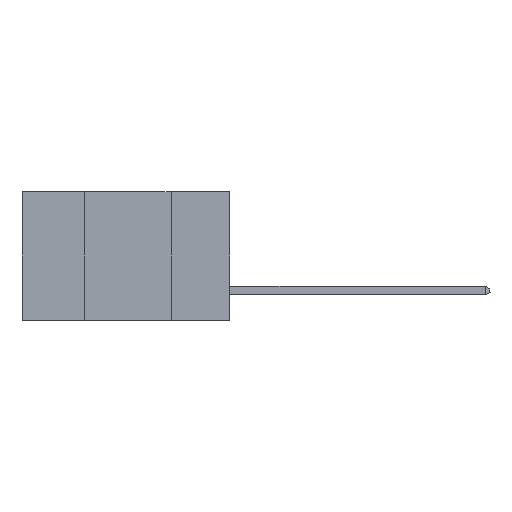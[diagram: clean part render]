
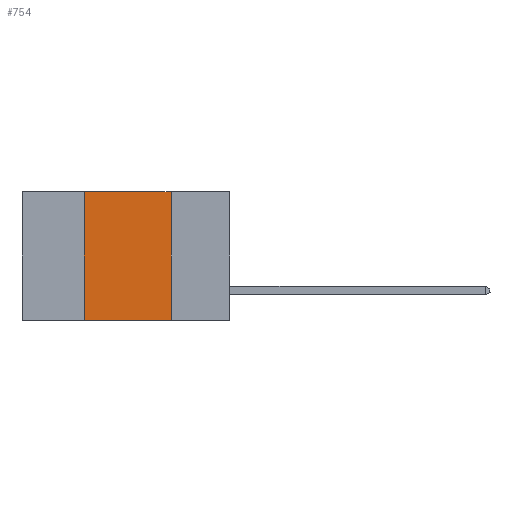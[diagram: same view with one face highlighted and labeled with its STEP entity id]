
A CAD part, left-side view. The second image highlights one B-rep face of the part: STEP entity #754.
In plain terms, the highlighted planar face has unit normal (-1, 0, 0).
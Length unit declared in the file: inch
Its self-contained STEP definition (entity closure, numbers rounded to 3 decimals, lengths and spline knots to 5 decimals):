
#754 = ADVANCED_FACE ( 'NONE', ( #15377 ), #8433, .F. ) ;
#2113 = VECTOR ( 'NONE', #14111, 39.37008 ) ;
#2684 = DIRECTION ( 'NONE',  ( 0., 0., 1. ) ) ;
#4161 = CARTESIAN_POINT ( 'NONE',  ( 0., 0.6, -0.37 ) ) ;
#4231 = CARTESIAN_POINT ( 'NONE',  ( 0., 0.42, 0. ) ) ;
#4242 = LINE ( 'NONE', #9874, #2113 ) ;
#4556 = DIRECTION ( 'NONE',  ( 0., 0., -1. ) ) ;
#5017 = ORIENTED_EDGE ( 'NONE', *, *, #5568, .F. ) ;
#5330 = ORIENTED_EDGE ( 'NONE', *, *, #8817, .F. ) ;
#5568 = EDGE_CURVE ( 'NONE', #24593, #8325, #8588, .T. ) ;
#6742 = DIRECTION ( 'NONE',  ( 1., 0., 0. ) ) ;
#8325 = VERTEX_POINT ( 'NONE', #4231 ) ;
#8433 = PLANE ( 'NONE',  #16339 ) ;
#8588 = LINE ( 'NONE', #8654, #13114 ) ;
#8654 = CARTESIAN_POINT ( 'NONE',  ( 0., 0.42, 0. ) ) ;
#8679 = CARTESIAN_POINT ( 'NONE',  ( 0., 0.6, 0. ) ) ;
#8817 = EDGE_CURVE ( 'NONE', #24569, #12203, #13921, .T. ) ;
#9874 = CARTESIAN_POINT ( 'NONE',  ( 0., 0.6, 0. ) ) ;
#10354 = VECTOR ( 'NONE', #14090, 39.37008 ) ;
#11654 = CARTESIAN_POINT ( 'NONE',  ( 0., 0.17, 0. ) ) ;
#12203 = VERTEX_POINT ( 'NONE', #24895 ) ;
#12506 = ORIENTED_EDGE ( 'NONE', *, *, #19374, .T. ) ;
#13114 = VECTOR ( 'NONE', #2684, 39.37008 ) ;
#13144 = EDGE_LOOP ( 'NONE', ( #5330, #22034, #5017, #12506 ) ) ;
#13921 = LINE ( 'NONE', #11654, #17844 ) ;
#14090 = DIRECTION ( 'NONE',  ( 0., -1., 0. ) ) ;
#14111 = DIRECTION ( 'NONE',  ( 0., -1., 0. ) ) ;
#14818 = CARTESIAN_POINT ( 'NONE',  ( 0., 0.17, 0. ) ) ;
#15377 = FACE_OUTER_BOUND ( 'NONE', #13144, .T. ) ;
#16339 = AXIS2_PLACEMENT_3D ( 'NONE', #8679, #6742, #4556 ) ;
#17844 = VECTOR ( 'NONE', #22907, 39.37008 ) ;
#19374 = EDGE_CURVE ( 'NONE', #24593, #12203, #20639, .T. ) ;
#20002 = EDGE_CURVE ( 'NONE', #8325, #24569, #4242, .T. ) ;
#20639 = LINE ( 'NONE', #4161, #10354 ) ;
#22034 = ORIENTED_EDGE ( 'NONE', *, *, #20002, .F. ) ;
#22907 = DIRECTION ( 'NONE',  ( 0., 0., -1. ) ) ;
#24429 = CARTESIAN_POINT ( 'NONE',  ( 0., 0.42, -0.37 ) ) ;
#24569 = VERTEX_POINT ( 'NONE', #14818 ) ;
#24593 = VERTEX_POINT ( 'NONE', #24429 ) ;
#24895 = CARTESIAN_POINT ( 'NONE',  ( 0., 0.17, -0.37 ) ) ;
